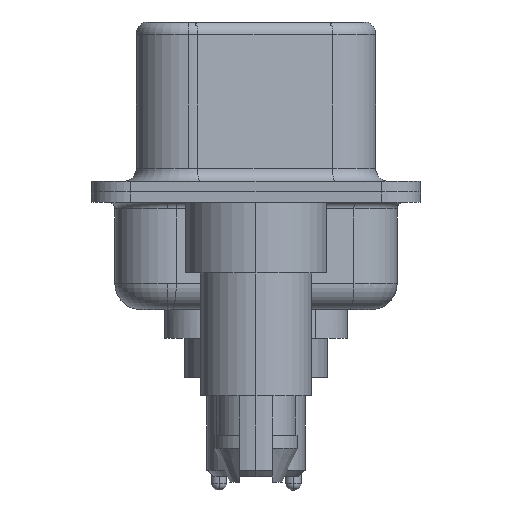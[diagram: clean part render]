
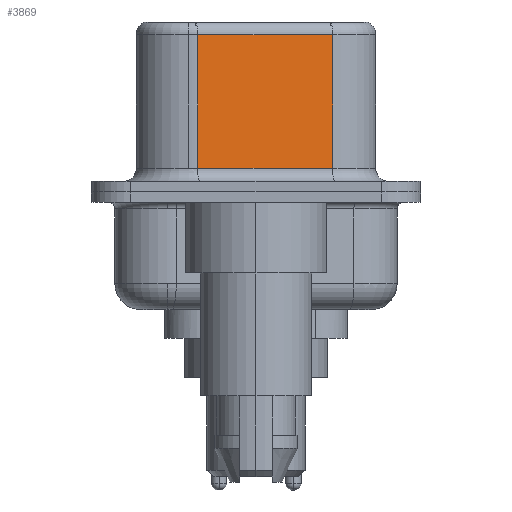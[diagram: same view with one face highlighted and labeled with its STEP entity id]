
A CAD part, left-side view. The second image highlights one B-rep face of the part: STEP entity #3869.
In plain terms, the highlighted planar face has unit normal (-0.985, -0.174, 0).
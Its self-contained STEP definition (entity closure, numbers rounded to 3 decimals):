
#29 = EDGE_CURVE ( 'NONE', #12732, #5145, #8617, .T. ) ;
#163 = VERTEX_POINT ( 'NONE', #18823 ) ;
#779 = VECTOR ( 'NONE', #13309, 1000. ) ;
#1038 = DIRECTION ( 'NONE',  ( 0.985, 0.174, 0. ) ) ;
#2609 = AXIS2_PLACEMENT_3D ( 'NONE', #11313, #1038, #16439 ) ;
#2785 = ORIENTED_EDGE ( 'NONE', *, *, #14740, .T. ) ;
#3132 = EDGE_LOOP ( 'NONE', ( #6785, #13053, #2785, #11467 ) ) ;
#3869 = ADVANCED_FACE ( 'NONE', ( #8644 ), #13259, .F. ) ;
#4764 = VECTOR ( 'NONE', #8428, 1000. ) ;
#4913 = VECTOR ( 'NONE', #5398, 1000. ) ;
#5093 = CARTESIAN_POINT ( 'NONE',  ( 4.58, -2.927, 6.02 ) ) ;
#5145 = VERTEX_POINT ( 'NONE', #15917 ) ;
#5244 = LINE ( 'NONE', #13156, #4764 ) ;
#5398 = DIRECTION ( 'NONE',  ( 0.174, -0.985, 0. ) ) ;
#5668 = CARTESIAN_POINT ( 'NONE',  ( 3.67, 2.233, 6.02 ) ) ;
#6175 = CARTESIAN_POINT ( 'NONE',  ( 4.58, -2.927, 0.9 ) ) ;
#6221 = EDGE_CURVE ( 'NONE', #163, #19341, #18992, .T. ) ;
#6502 = CARTESIAN_POINT ( 'NONE',  ( 3.67, 2.233, 0.9 ) ) ;
#6785 = ORIENTED_EDGE ( 'NONE', *, *, #19280, .F. ) ;
#8428 = DIRECTION ( 'NONE',  ( 0., 0., -1. ) ) ;
#8617 = LINE ( 'NONE', #6175, #4913 ) ;
#8644 = FACE_OUTER_BOUND ( 'NONE', #3132, .T. ) ;
#11313 = CARTESIAN_POINT ( 'NONE',  ( 4.58, -2.927, 6.52 ) ) ;
#11467 = ORIENTED_EDGE ( 'NONE', *, *, #29, .T. ) ;
#11691 = VECTOR ( 'NONE', #13831, 1000. ) ;
#11739 = CARTESIAN_POINT ( 'NONE',  ( 4.58, -2.927, 6.52 ) ) ;
#12716 = LINE ( 'NONE', #11739, #779 ) ;
#12732 = VERTEX_POINT ( 'NONE', #6502 ) ;
#13053 = ORIENTED_EDGE ( 'NONE', *, *, #6221, .T. ) ;
#13156 = CARTESIAN_POINT ( 'NONE',  ( 3.67, 2.233, 6.52 ) ) ;
#13259 = PLANE ( 'NONE',  #2609 ) ;
#13309 = DIRECTION ( 'NONE',  ( 0., 0., -1. ) ) ;
#13831 = DIRECTION ( 'NONE',  ( -0.174, 0.985, 0. ) ) ;
#14740 = EDGE_CURVE ( 'NONE', #19341, #12732, #5244, .T. ) ;
#15917 = CARTESIAN_POINT ( 'NONE',  ( 4.58, -2.927, 0.9 ) ) ;
#16439 = DIRECTION ( 'NONE',  ( -0.174, 0.985, 0. ) ) ;
#18823 = CARTESIAN_POINT ( 'NONE',  ( 4.58, -2.927, 6.02 ) ) ;
#18992 = LINE ( 'NONE', #5093, #11691 ) ;
#19280 = EDGE_CURVE ( 'NONE', #163, #5145, #12716, .T. ) ;
#19341 = VERTEX_POINT ( 'NONE', #5668 ) ;
